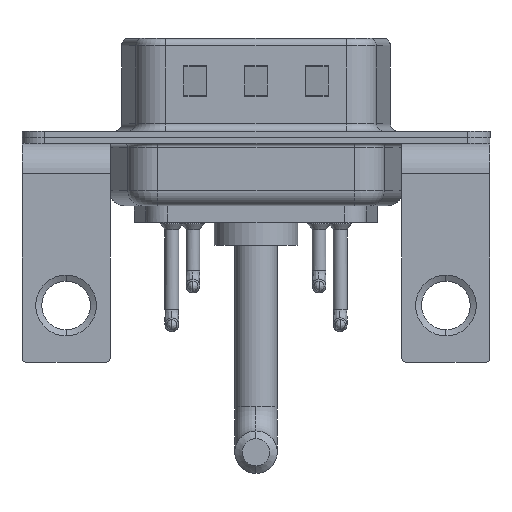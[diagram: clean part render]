
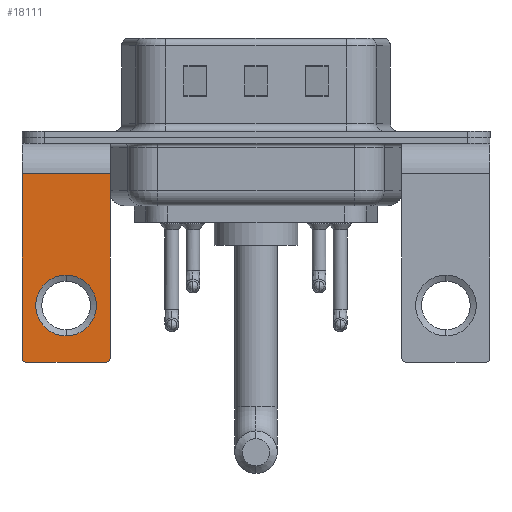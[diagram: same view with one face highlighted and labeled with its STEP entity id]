
A CAD part, front view. The second image highlights one B-rep face of the part: STEP entity #18111.
In plain terms, the highlighted planar face has unit normal (0, -1, 0).
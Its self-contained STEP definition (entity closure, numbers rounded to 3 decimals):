
#195 = DIRECTION ( 'NONE',  ( 0., 0., 1. ) ) ;
#439 = VERTEX_POINT ( 'NONE', #17944 ) ;
#775 = CARTESIAN_POINT ( 'NONE',  ( -2.9, -6.25, -2.4 ) ) ;
#1124 = EDGE_CURVE ( 'NONE', #4120, #4274, #13998, .T. ) ;
#1253 = FACE_OUTER_BOUND ( 'NONE', #1351, .T. ) ;
#1302 = CIRCLE ( 'NONE', #12686, 0.25 ) ;
#1314 = CARTESIAN_POINT ( 'NONE',  ( 0., -6.25, -11.07 ) ) ;
#1351 = EDGE_LOOP ( 'NONE', ( #12165, #7450, #3511, #14848, #9760, #8275 ) ) ;
#1687 = CARTESIAN_POINT ( 'NONE',  ( 2.65, -6.25, -14.8 ) ) ;
#1769 = LINE ( 'NONE', #3384, #15235 ) ;
#2050 = CARTESIAN_POINT ( 'NONE',  ( 0., -6.25, -13.07 ) ) ;
#2148 = DIRECTION ( 'NONE',  ( 0., 0., -1. ) ) ;
#3214 = VECTOR ( 'NONE', #15275, 1000. ) ;
#3384 = CARTESIAN_POINT ( 'NONE',  ( 2.9, -6.25, -2.4 ) ) ;
#3511 = ORIENTED_EDGE ( 'NONE', *, *, #9898, .F. ) ;
#3692 = DIRECTION ( 'NONE',  ( 0., 0., 1. ) ) ;
#3987 = ORIENTED_EDGE ( 'NONE', *, *, #1124, .T. ) ;
#4003 = CIRCLE ( 'NONE', #15379, 2. ) ;
#4111 = LINE ( 'NONE', #8810, #11653 ) ;
#4120 = VERTEX_POINT ( 'NONE', #2050 ) ;
#4274 = VERTEX_POINT ( 'NONE', #7241 ) ;
#4514 = FACE_BOUND ( 'NONE', #8255, .T. ) ;
#4738 = VERTEX_POINT ( 'NONE', #1687 ) ;
#4974 = VERTEX_POINT ( 'NONE', #775 ) ;
#5080 = DIRECTION ( 'NONE',  ( 0., 1., 0. ) ) ;
#5447 = EDGE_CURVE ( 'NONE', #4738, #19877, #1302, .T. ) ;
#6296 = CARTESIAN_POINT ( 'NONE',  ( 2.9, -6.25, -14.55 ) ) ;
#6341 = CARTESIAN_POINT ( 'NONE',  ( -2.9, -6.25, -2.4 ) ) ;
#6560 = EDGE_CURVE ( 'NONE', #439, #16752, #19846, .T. ) ;
#7134 = VERTEX_POINT ( 'NONE', #17696 ) ;
#7241 = CARTESIAN_POINT ( 'NONE',  ( 0., -6.25, -9.07 ) ) ;
#7450 = ORIENTED_EDGE ( 'NONE', *, *, #6560, .T. ) ;
#7470 = DIRECTION ( 'NONE',  ( 0., 1., 0. ) ) ;
#7772 = CARTESIAN_POINT ( 'NONE',  ( 2.9, -6.25, -2.4 ) ) ;
#8079 = VECTOR ( 'NONE', #9389, 1000. ) ;
#8145 = AXIS2_PLACEMENT_3D ( 'NONE', #19013, #5080, #195 ) ;
#8255 = EDGE_LOOP ( 'NONE', ( #3987, #17035 ) ) ;
#8275 = ORIENTED_EDGE ( 'NONE', *, *, #14049, .T. ) ;
#8810 = CARTESIAN_POINT ( 'NONE',  ( 2.9, -6.25, -14.8 ) ) ;
#9344 = DIRECTION ( 'NONE',  ( 0., 0., 1. ) ) ;
#9389 = DIRECTION ( 'NONE',  ( 0., 0., -1. ) ) ;
#9692 = EDGE_CURVE ( 'NONE', #4274, #4120, #4003, .T. ) ;
#9760 = ORIENTED_EDGE ( 'NONE', *, *, #10134, .F. ) ;
#9802 = LINE ( 'NONE', #6341, #8079 ) ;
#9898 = EDGE_CURVE ( 'NONE', #4738, #16752, #4111, .T. ) ;
#10134 = EDGE_CURVE ( 'NONE', #7134, #19877, #1769, .T. ) ;
#10679 = LINE ( 'NONE', #15386, #3214 ) ;
#10715 = PLANE ( 'NONE',  #11678 ) ;
#10871 = DIRECTION ( 'NONE',  ( 0., 1., 0. ) ) ;
#11087 = AXIS2_PLACEMENT_3D ( 'NONE', #14190, #15731, #3692 ) ;
#11653 = VECTOR ( 'NONE', #12151, 1000. ) ;
#11678 = AXIS2_PLACEMENT_3D ( 'NONE', #7772, #7470, #15414 ) ;
#12151 = DIRECTION ( 'NONE',  ( -1., 0., 0. ) ) ;
#12165 = ORIENTED_EDGE ( 'NONE', *, *, #16768, .T. ) ;
#12686 = AXIS2_PLACEMENT_3D ( 'NONE', #18905, #14035, #18489 ) ;
#13998 = CIRCLE ( 'NONE', #8145, 2. ) ;
#14035 = DIRECTION ( 'NONE',  ( 0., -1., 0. ) ) ;
#14049 = EDGE_CURVE ( 'NONE', #7134, #4974, #10679, .T. ) ;
#14190 = CARTESIAN_POINT ( 'NONE',  ( -2.65, -6.25, -14.55 ) ) ;
#14848 = ORIENTED_EDGE ( 'NONE', *, *, #5447, .T. ) ;
#15235 = VECTOR ( 'NONE', #2148, 1000. ) ;
#15275 = DIRECTION ( 'NONE',  ( -1., 0., 0. ) ) ;
#15379 = AXIS2_PLACEMENT_3D ( 'NONE', #1314, #10871, #9344 ) ;
#15386 = CARTESIAN_POINT ( 'NONE',  ( 2.9, -6.25, -2.4 ) ) ;
#15414 = DIRECTION ( 'NONE',  ( 0., 0., 1. ) ) ;
#15731 = DIRECTION ( 'NONE',  ( 0., -1., 0. ) ) ;
#16021 = CARTESIAN_POINT ( 'NONE',  ( -2.65, -6.25, -14.8 ) ) ;
#16752 = VERTEX_POINT ( 'NONE', #16021 ) ;
#16768 = EDGE_CURVE ( 'NONE', #4974, #439, #9802, .T. ) ;
#17035 = ORIENTED_EDGE ( 'NONE', *, *, #9692, .T. ) ;
#17696 = CARTESIAN_POINT ( 'NONE',  ( 2.9, -6.25, -2.4 ) ) ;
#17944 = CARTESIAN_POINT ( 'NONE',  ( -2.9, -6.25, -14.55 ) ) ;
#18111 = ADVANCED_FACE ( 'NONE', ( #4514, #1253 ), #10715, .F. ) ;
#18489 = DIRECTION ( 'NONE',  ( 0., 0., 1. ) ) ;
#18905 = CARTESIAN_POINT ( 'NONE',  ( 2.65, -6.25, -14.55 ) ) ;
#19013 = CARTESIAN_POINT ( 'NONE',  ( 0., -6.25, -11.07 ) ) ;
#19846 = CIRCLE ( 'NONE', #11087, 0.25 ) ;
#19877 = VERTEX_POINT ( 'NONE', #6296 ) ;
